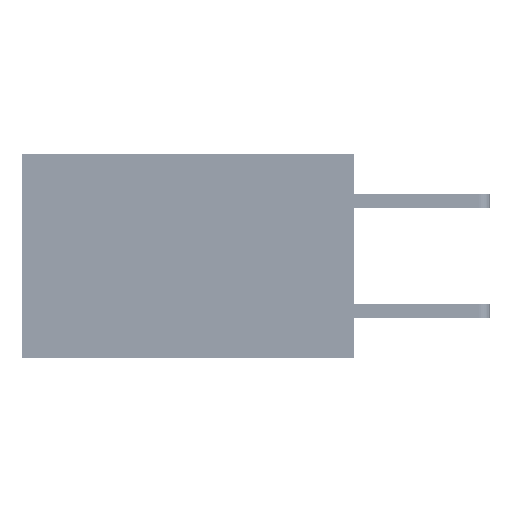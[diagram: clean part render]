
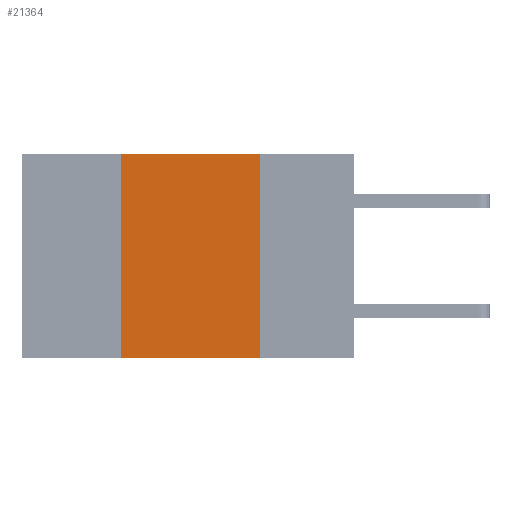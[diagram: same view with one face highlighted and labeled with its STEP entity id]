
A CAD part, left-side view. The second image highlights one B-rep face of the part: STEP entity #21364.
In plain terms, the highlighted planar face has unit normal (-1, 0, 0).
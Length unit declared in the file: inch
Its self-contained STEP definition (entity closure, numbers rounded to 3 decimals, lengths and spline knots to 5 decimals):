
#338 = VERTEX_POINT ( 'NONE', #25746 ) ;
#1273 = DIRECTION ( 'NONE',  ( 0., -1., 0. ) ) ;
#1748 = LINE ( 'NONE', #9218, #31238 ) ;
#3928 = DIRECTION ( 'NONE',  ( 0., 0., 1. ) ) ;
#5746 = DIRECTION ( 'NONE',  ( 0., 0., -1. ) ) ;
#7926 = ORIENTED_EDGE ( 'NONE', *, *, #31885, .F. ) ;
#9218 = CARTESIAN_POINT ( 'NONE',  ( 0., 0.17, 0. ) ) ;
#14364 = DIRECTION ( 'NONE',  ( 0., -1., 0. ) ) ;
#14372 = LINE ( 'NONE', #18827, #17299 ) ;
#15104 = LINE ( 'NONE', #18079, #30046 ) ;
#15517 = ORIENTED_EDGE ( 'NONE', *, *, #33205, .F. ) ;
#17299 = VECTOR ( 'NONE', #3928, 39.37008 ) ;
#17470 = ORIENTED_EDGE ( 'NONE', *, *, #25910, .F. ) ;
#18079 = CARTESIAN_POINT ( 'NONE',  ( 0., 0.6, 0. ) ) ;
#18827 = CARTESIAN_POINT ( 'NONE',  ( 0., 0.42, 0. ) ) ;
#20175 = LINE ( 'NONE', #35112, #37000 ) ;
#20548 = PLANE ( 'NONE',  #23836 ) ;
#21364 = ADVANCED_FACE ( 'NONE', ( #24996 ), #20548, .F. ) ;
#22351 = VERTEX_POINT ( 'NONE', #32847 ) ;
#23836 = AXIS2_PLACEMENT_3D ( 'NONE', #47363, #47126, #39674 ) ;
#24996 = FACE_OUTER_BOUND ( 'NONE', #40726, .T. ) ;
#25746 = CARTESIAN_POINT ( 'NONE',  ( 0., 0.42, 0. ) ) ;
#25910 = EDGE_CURVE ( 'NONE', #22351, #41837, #1748, .T. ) ;
#29164 = EDGE_CURVE ( 'NONE', #48178, #41837, #20175, .T. ) ;
#29204 = CARTESIAN_POINT ( 'NONE',  ( 0., 0.42, -0.37 ) ) ;
#30046 = VECTOR ( 'NONE', #14364, 39.37008 ) ;
#31238 = VECTOR ( 'NONE', #5746, 39.37008 ) ;
#31885 = EDGE_CURVE ( 'NONE', #338, #22351, #15104, .T. ) ;
#32416 = CARTESIAN_POINT ( 'NONE',  ( 0., 0.17, -0.37 ) ) ;
#32847 = CARTESIAN_POINT ( 'NONE',  ( 0., 0.17, 0. ) ) ;
#33205 = EDGE_CURVE ( 'NONE', #48178, #338, #14372, .T. ) ;
#35112 = CARTESIAN_POINT ( 'NONE',  ( 0., 0.6, -0.37 ) ) ;
#36850 = ORIENTED_EDGE ( 'NONE', *, *, #29164, .T. ) ;
#37000 = VECTOR ( 'NONE', #1273, 39.37008 ) ;
#39674 = DIRECTION ( 'NONE',  ( 0., 0., -1. ) ) ;
#40726 = EDGE_LOOP ( 'NONE', ( #17470, #7926, #15517, #36850 ) ) ;
#41837 = VERTEX_POINT ( 'NONE', #32416 ) ;
#47126 = DIRECTION ( 'NONE',  ( 1., 0., 0. ) ) ;
#47363 = CARTESIAN_POINT ( 'NONE',  ( 0., 0.6, 0. ) ) ;
#48178 = VERTEX_POINT ( 'NONE', #29204 ) ;
